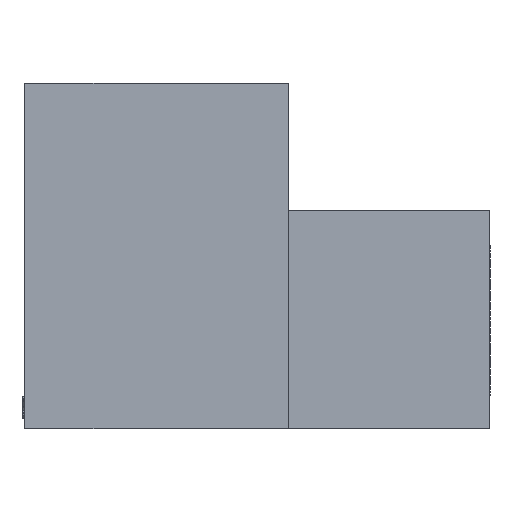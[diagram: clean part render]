
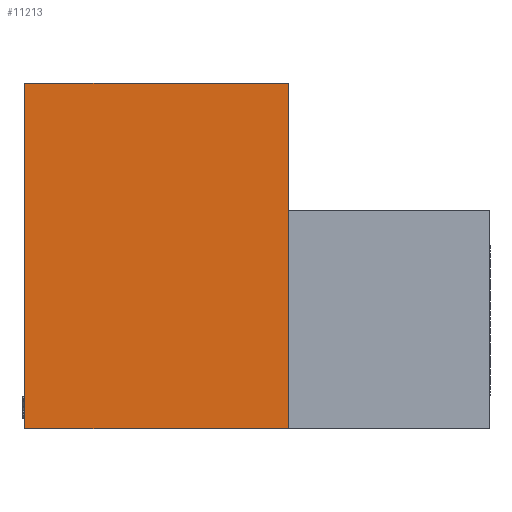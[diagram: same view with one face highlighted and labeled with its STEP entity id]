
A CAD part, left-side view. The second image highlights one B-rep face of the part: STEP entity #11213.
In plain terms, the highlighted planar face has unit normal (-1, 0, 0).
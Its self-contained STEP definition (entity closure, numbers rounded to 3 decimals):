
#691 = LINE ( 'NONE', #19570, #22306 ) ;
#2355 = ORIENTED_EDGE ( 'NONE', *, *, #43543, .F. ) ;
#2457 = DIRECTION ( 'NONE',  ( 0., -1., 0. ) ) ;
#3963 = ORIENTED_EDGE ( 'NONE', *, *, #15789, .F. ) ;
#8486 = CARTESIAN_POINT ( 'NONE',  ( 0., 0., 0. ) ) ;
#8886 = LINE ( 'NONE', #31822, #42959 ) ;
#11213 = ADVANCED_FACE ( 'NONE', ( #34901 ), #43192, .F. ) ;
#11503 = VECTOR ( 'NONE', #31532, 1000. ) ;
#12393 = DIRECTION ( 'NONE',  ( 0., 1., 0. ) ) ;
#13922 = AXIS2_PLACEMENT_3D ( 'NONE', #42573, #46856, #21181 ) ;
#15292 = CARTESIAN_POINT ( 'NONE',  ( 0., 0., 0. ) ) ;
#15789 = EDGE_CURVE ( 'NONE', #38026, #24318, #17193, .T. ) ;
#17193 = LINE ( 'NONE', #45946, #11503 ) ;
#19570 = CARTESIAN_POINT ( 'NONE',  ( 0., -8.814, -15.088 ) ) ;
#20716 = EDGE_LOOP ( 'NONE', ( #28967, #39710, #2355, #3963 ) ) ;
#20720 = CARTESIAN_POINT ( 'NONE',  ( 0., 11.506, -15.088 ) ) ;
#21181 = DIRECTION ( 'NONE',  ( 0., 0., -1. ) ) ;
#22306 = VECTOR ( 'NONE', #12393, 1000. ) ;
#24318 = VERTEX_POINT ( 'NONE', #38517 ) ;
#27837 = EDGE_CURVE ( 'NONE', #42979, #36853, #31475, .T. ) ;
#28967 = ORIENTED_EDGE ( 'NONE', *, *, #32362, .F. ) ;
#31475 = LINE ( 'NONE', #8486, #37161 ) ;
#31532 = DIRECTION ( 'NONE',  ( 0., 0., 1. ) ) ;
#31822 = CARTESIAN_POINT ( 'NONE',  ( 0., 11.506, 0. ) ) ;
#32362 = EDGE_CURVE ( 'NONE', #36853, #38026, #691, .T. ) ;
#34901 = FACE_OUTER_BOUND ( 'NONE', #20716, .T. ) ;
#36853 = VERTEX_POINT ( 'NONE', #45028 ) ;
#37161 = VECTOR ( 'NONE', #45627, 1000. ) ;
#38026 = VERTEX_POINT ( 'NONE', #20720 ) ;
#38517 = CARTESIAN_POINT ( 'NONE',  ( 0., 11.506, 0. ) ) ;
#39710 = ORIENTED_EDGE ( 'NONE', *, *, #27837, .F. ) ;
#42573 = CARTESIAN_POINT ( 'NONE',  ( 0., 0., 0. ) ) ;
#42959 = VECTOR ( 'NONE', #2457, 1000. ) ;
#42979 = VERTEX_POINT ( 'NONE', #15292 ) ;
#43192 = PLANE ( 'NONE',  #13922 ) ;
#43543 = EDGE_CURVE ( 'NONE', #24318, #42979, #8886, .T. ) ;
#45028 = CARTESIAN_POINT ( 'NONE',  ( 0., 0., -15.088 ) ) ;
#45627 = DIRECTION ( 'NONE',  ( 0., 0., -1. ) ) ;
#45946 = CARTESIAN_POINT ( 'NONE',  ( 0., 11.506, -15.088 ) ) ;
#46856 = DIRECTION ( 'NONE',  ( 1., 0., 0. ) ) ;
